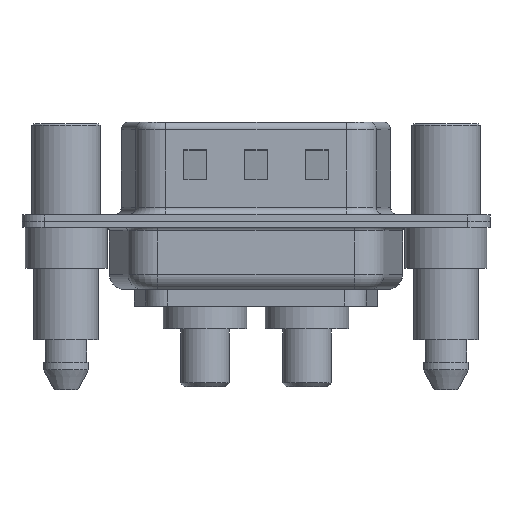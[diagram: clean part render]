
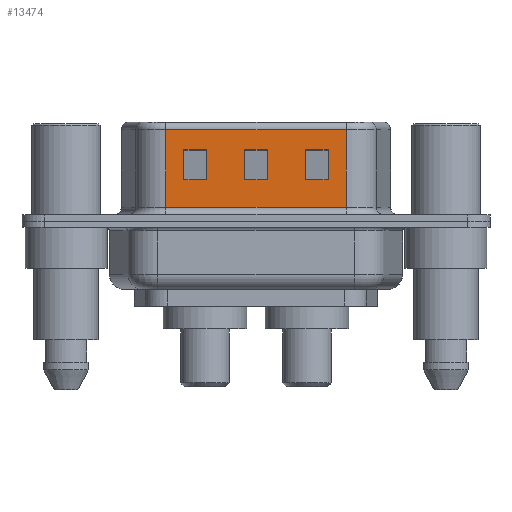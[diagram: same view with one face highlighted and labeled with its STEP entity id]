
A CAD part, front view. The second image highlights one B-rep face of the part: STEP entity #13474.
In plain terms, the highlighted planar face has unit normal (0, -1, 0).
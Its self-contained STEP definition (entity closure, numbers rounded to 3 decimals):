
#76 = VERTEX_POINT ( 'NONE', #677 ) ;
#93 = CARTESIAN_POINT ( 'NONE',  ( 13.25, -4.58, 6.52 ) ) ;
#677 = CARTESIAN_POINT ( 'NONE',  ( 9.25, -4.58, 2.705 ) ) ;
#725 = FACE_BOUND ( 'NONE', #8810, .T. ) ;
#1182 = FACE_OUTER_BOUND ( 'NONE', #3514, .T. ) ;
#1213 = ORIENTED_EDGE ( 'NONE', *, *, #14682, .T. ) ;
#1243 = LINE ( 'NONE', #12459, #7935 ) ;
#1449 = VERTEX_POINT ( 'NONE', #14766 ) ;
#1459 = VECTOR ( 'NONE', #2024, 1000. ) ;
#1567 = CARTESIAN_POINT ( 'NONE',  ( 18.45, -4.58, 0.9 ) ) ;
#1568 = DIRECTION ( 'NONE',  ( -1., 0., 0. ) ) ;
#1630 = CARTESIAN_POINT ( 'NONE',  ( 9.25, -4.58, 4.705 ) ) ;
#1714 = VECTOR ( 'NONE', #3122, 1000. ) ;
#1846 = VERTEX_POINT ( 'NONE', #6098 ) ;
#1960 = CARTESIAN_POINT ( 'NONE',  ( 14.45, -4.58, 4.705 ) ) ;
#2024 = DIRECTION ( 'NONE',  ( 1., 0., 0. ) ) ;
#2053 = LINE ( 'NONE', #14661, #16168 ) ;
#2196 = LINE ( 'NONE', #7384, #1714 ) ;
#2887 = ORIENTED_EDGE ( 'NONE', *, *, #6133, .T. ) ;
#3122 = DIRECTION ( 'NONE',  ( 0., 0., -1. ) ) ;
#3195 = ORIENTED_EDGE ( 'NONE', *, *, #5069, .T. ) ;
#3227 = CARTESIAN_POINT ( 'NONE',  ( 17.25, -4.58, 6.52 ) ) ;
#3423 = AXIS2_PLACEMENT_3D ( 'NONE', #8387, #7071, #16423 ) ;
#3514 = EDGE_LOOP ( 'NONE', ( #9740, #11359, #14373, #9621 ) ) ;
#3519 = VERTEX_POINT ( 'NONE', #1630 ) ;
#3637 = VECTOR ( 'NONE', #6920, 1000. ) ;
#3780 = VECTOR ( 'NONE', #8703, 1000. ) ;
#4091 = ORIENTED_EDGE ( 'NONE', *, *, #6913, .T. ) ;
#4111 = ORIENTED_EDGE ( 'NONE', *, *, #16055, .T. ) ;
#4188 = EDGE_CURVE ( 'NONE', #9214, #12939, #10218, .T. ) ;
#4520 = FACE_BOUND ( 'NONE', #8780, .T. ) ;
#4542 = DIRECTION ( 'NONE',  ( -1., 0., 0. ) ) ;
#4671 = LINE ( 'NONE', #14981, #12047 ) ;
#5069 = EDGE_CURVE ( 'NONE', #12939, #13681, #8261, .T. ) ;
#5206 = LINE ( 'NONE', #6601, #15188 ) ;
#5245 = ORIENTED_EDGE ( 'NONE', *, *, #11013, .T. ) ;
#5277 = LINE ( 'NONE', #15601, #15269 ) ;
#5412 = EDGE_CURVE ( 'NONE', #10196, #10951, #2053, .T. ) ;
#5603 = ORIENTED_EDGE ( 'NONE', *, *, #7870, .T. ) ;
#5673 = EDGE_CURVE ( 'NONE', #8605, #9399, #4671, .T. ) ;
#5815 = CARTESIAN_POINT ( 'NONE',  ( 6.55, -4.58, 0.9 ) ) ;
#6049 = VECTOR ( 'NONE', #15606, 1000. ) ;
#6098 = CARTESIAN_POINT ( 'NONE',  ( 17.25, -4.58, 4.705 ) ) ;
#6133 = EDGE_CURVE ( 'NONE', #13681, #10991, #14675, .T. ) ;
#6241 = VERTEX_POINT ( 'NONE', #6746 ) ;
#6601 = CARTESIAN_POINT ( 'NONE',  ( 15.75, -4.58, 6.52 ) ) ;
#6635 = VERTEX_POINT ( 'NONE', #15832 ) ;
#6646 = ORIENTED_EDGE ( 'NONE', *, *, #9958, .T. ) ;
#6692 = DIRECTION ( 'NONE',  ( 1., 0., 0. ) ) ;
#6746 = CARTESIAN_POINT ( 'NONE',  ( 6.55, -4.58, 6.02 ) ) ;
#6913 = EDGE_CURVE ( 'NONE', #76, #6635, #5277, .T. ) ;
#6920 = DIRECTION ( 'NONE',  ( 1., 0., 0. ) ) ;
#7071 = DIRECTION ( 'NONE',  ( 0., 1., 0. ) ) ;
#7384 = CARTESIAN_POINT ( 'NONE',  ( 6.55, -4.58, 6.52 ) ) ;
#7502 = LINE ( 'NONE', #13993, #3780 ) ;
#7870 = EDGE_CURVE ( 'NONE', #3519, #76, #9878, .T. ) ;
#7935 = VECTOR ( 'NONE', #12770, 1000. ) ;
#8092 = ORIENTED_EDGE ( 'NONE', *, *, #10150, .T. ) ;
#8255 = LINE ( 'NONE', #14928, #14915 ) ;
#8261 = LINE ( 'NONE', #13574, #14917 ) ;
#8387 = CARTESIAN_POINT ( 'NONE',  ( 18.45, -4.58, 6.52 ) ) ;
#8428 = ORIENTED_EDGE ( 'NONE', *, *, #17061, .T. ) ;
#8431 = VECTOR ( 'NONE', #14933, 1000. ) ;
#8605 = VERTEX_POINT ( 'NONE', #17136 ) ;
#8703 = DIRECTION ( 'NONE',  ( -1., 0., 0. ) ) ;
#8780 = EDGE_LOOP ( 'NONE', ( #5603, #4091, #8092, #8428 ) ) ;
#8810 = EDGE_LOOP ( 'NONE', ( #3195, #2887, #1213, #10563 ) ) ;
#8865 = CARTESIAN_POINT ( 'NONE',  ( 13.25, -4.58, 4.705 ) ) ;
#8874 = LINE ( 'NONE', #1567, #15951 ) ;
#9214 = VERTEX_POINT ( 'NONE', #15542 ) ;
#9399 = VERTEX_POINT ( 'NONE', #15414 ) ;
#9456 = VECTOR ( 'NONE', #10238, 1000. ) ;
#9476 = CARTESIAN_POINT ( 'NONE',  ( 11.75, -4.58, 6.52 ) ) ;
#9609 = EDGE_CURVE ( 'NONE', #6241, #13582, #2196, .T. ) ;
#9621 = ORIENTED_EDGE ( 'NONE', *, *, #15612, .T. ) ;
#9740 = ORIENTED_EDGE ( 'NONE', *, *, #5673, .F. ) ;
#9878 = LINE ( 'NONE', #14879, #9456 ) ;
#9958 = EDGE_CURVE ( 'NONE', #1846, #10196, #10899, .T. ) ;
#10150 = EDGE_CURVE ( 'NONE', #6635, #14445, #1243, .T. ) ;
#10196 = VERTEX_POINT ( 'NONE', #10818 ) ;
#10218 = LINE ( 'NONE', #9476, #6049 ) ;
#10238 = DIRECTION ( 'NONE',  ( 0., 0., -1. ) ) ;
#10563 = ORIENTED_EDGE ( 'NONE', *, *, #4188, .T. ) ;
#10818 = CARTESIAN_POINT ( 'NONE',  ( 17.25, -4.58, 2.705 ) ) ;
#10899 = LINE ( 'NONE', #3227, #14402 ) ;
#10951 = VERTEX_POINT ( 'NONE', #17243 ) ;
#10991 = VERTEX_POINT ( 'NONE', #13276 ) ;
#11013 = EDGE_CURVE ( 'NONE', #10951, #1449, #5206, .T. ) ;
#11071 = CARTESIAN_POINT ( 'NONE',  ( 11.75, -4.58, 4.705 ) ) ;
#11281 = DIRECTION ( 'NONE',  ( 1., 0., 0. ) ) ;
#11359 = ORIENTED_EDGE ( 'NONE', *, *, #16872, .T. ) ;
#11390 = LINE ( 'NONE', #16284, #3637 ) ;
#11886 = FACE_BOUND ( 'NONE', #15344, .T. ) ;
#11919 = ORIENTED_EDGE ( 'NONE', *, *, #5412, .T. ) ;
#12047 = VECTOR ( 'NONE', #17297, 1000. ) ;
#12366 = DIRECTION ( 'NONE',  ( -1., 0., 0. ) ) ;
#12459 = CARTESIAN_POINT ( 'NONE',  ( 7.75, -4.58, 6.52 ) ) ;
#12570 = LINE ( 'NONE', #1960, #1459 ) ;
#12770 = DIRECTION ( 'NONE',  ( 0., 0., 1. ) ) ;
#12939 = VERTEX_POINT ( 'NONE', #11071 ) ;
#13276 = CARTESIAN_POINT ( 'NONE',  ( 13.25, -4.58, 2.705 ) ) ;
#13474 = ADVANCED_FACE ( 'NONE', ( #4520, #11886, #725, #1182 ), #15079, .F. ) ;
#13574 = CARTESIAN_POINT ( 'NONE',  ( 18.45, -4.58, 4.705 ) ) ;
#13582 = VERTEX_POINT ( 'NONE', #5815 ) ;
#13681 = VERTEX_POINT ( 'NONE', #8865 ) ;
#13993 = CARTESIAN_POINT ( 'NONE',  ( 18.45, -4.58, 6.02 ) ) ;
#14373 = ORIENTED_EDGE ( 'NONE', *, *, #9609, .T. ) ;
#14402 = VECTOR ( 'NONE', #17483, 1000. ) ;
#14445 = VERTEX_POINT ( 'NONE', #17302 ) ;
#14661 = CARTESIAN_POINT ( 'NONE',  ( 22.45, -4.58, 2.705 ) ) ;
#14675 = LINE ( 'NONE', #93, #8431 ) ;
#14682 = EDGE_CURVE ( 'NONE', #10991, #9214, #8255, .T. ) ;
#14766 = CARTESIAN_POINT ( 'NONE',  ( 15.75, -4.58, 4.705 ) ) ;
#14879 = CARTESIAN_POINT ( 'NONE',  ( 9.25, -4.58, 6.52 ) ) ;
#14915 = VECTOR ( 'NONE', #12366, 1000. ) ;
#14917 = VECTOR ( 'NONE', #6692, 1000. ) ;
#14928 = CARTESIAN_POINT ( 'NONE',  ( 18.45, -4.58, 2.705 ) ) ;
#14933 = DIRECTION ( 'NONE',  ( 0., 0., -1. ) ) ;
#14981 = CARTESIAN_POINT ( 'NONE',  ( 18.45, -4.58, 6.52 ) ) ;
#15079 = PLANE ( 'NONE',  #3423 ) ;
#15188 = VECTOR ( 'NONE', #17360, 1000. ) ;
#15269 = VECTOR ( 'NONE', #1568, 1000. ) ;
#15344 = EDGE_LOOP ( 'NONE', ( #6646, #11919, #5245, #4111 ) ) ;
#15414 = CARTESIAN_POINT ( 'NONE',  ( 18.45, -4.58, 0.9 ) ) ;
#15542 = CARTESIAN_POINT ( 'NONE',  ( 11.75, -4.58, 2.705 ) ) ;
#15601 = CARTESIAN_POINT ( 'NONE',  ( 14.45, -4.58, 2.705 ) ) ;
#15606 = DIRECTION ( 'NONE',  ( 0., 0., 1. ) ) ;
#15612 = EDGE_CURVE ( 'NONE', #13582, #9399, #8874, .T. ) ;
#15832 = CARTESIAN_POINT ( 'NONE',  ( 7.75, -4.58, 2.705 ) ) ;
#15951 = VECTOR ( 'NONE', #11281, 1000. ) ;
#16055 = EDGE_CURVE ( 'NONE', #1449, #1846, #11390, .T. ) ;
#16168 = VECTOR ( 'NONE', #4542, 1000. ) ;
#16284 = CARTESIAN_POINT ( 'NONE',  ( 22.45, -4.58, 4.705 ) ) ;
#16423 = DIRECTION ( 'NONE',  ( 0., 0., 1. ) ) ;
#16872 = EDGE_CURVE ( 'NONE', #8605, #6241, #7502, .T. ) ;
#17061 = EDGE_CURVE ( 'NONE', #14445, #3519, #12570, .T. ) ;
#17136 = CARTESIAN_POINT ( 'NONE',  ( 18.45, -4.58, 6.02 ) ) ;
#17243 = CARTESIAN_POINT ( 'NONE',  ( 15.75, -4.58, 2.705 ) ) ;
#17297 = DIRECTION ( 'NONE',  ( 0., 0., -1. ) ) ;
#17302 = CARTESIAN_POINT ( 'NONE',  ( 7.75, -4.58, 4.705 ) ) ;
#17360 = DIRECTION ( 'NONE',  ( 0., 0., 1. ) ) ;
#17483 = DIRECTION ( 'NONE',  ( 0., 0., -1. ) ) ;
